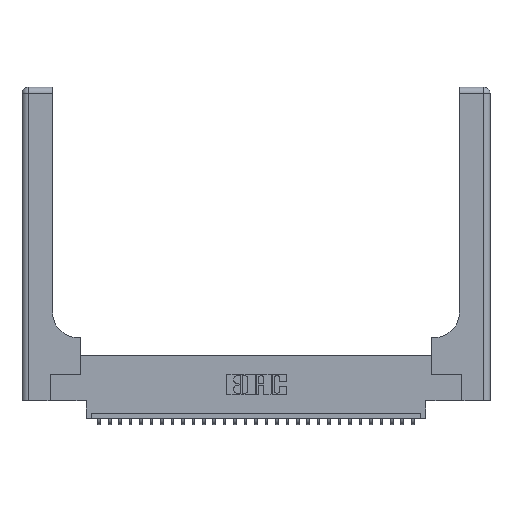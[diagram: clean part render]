
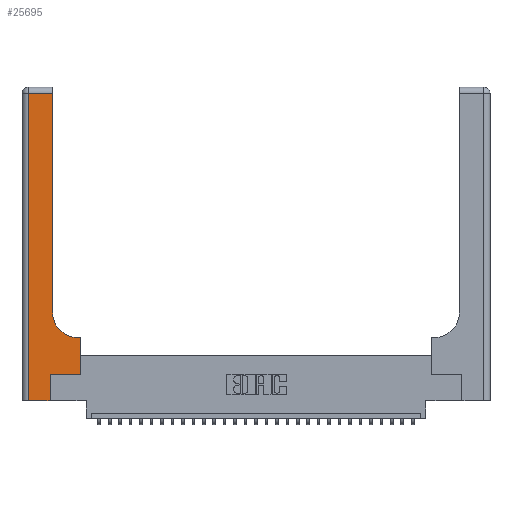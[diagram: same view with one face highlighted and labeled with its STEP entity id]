
A CAD part, top view. The second image highlights one B-rep face of the part: STEP entity #25695.
In plain terms, the highlighted planar face has unit normal (0, 0, 1).
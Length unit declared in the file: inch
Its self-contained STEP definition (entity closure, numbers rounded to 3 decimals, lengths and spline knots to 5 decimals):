
#50 = VERTEX_POINT ( 'NONE', #26670 ) ;
#305 = CARTESIAN_POINT ( 'NONE',  ( 0.5585, 0.6, 0.37 ) ) ;
#735 = LINE ( 'NONE', #1830, #29548 ) ;
#1077 = DIRECTION ( 'NONE',  ( -1., 0., 0. ) ) ;
#1157 = CARTESIAN_POINT ( 'NONE',  ( 0.269, 0., 0.37 ) ) ;
#1633 = CARTESIAN_POINT ( 'NONE',  ( 0.06, 3., 0.37 ) ) ;
#1830 = CARTESIAN_POINT ( 'NONE',  ( 0.2915, 3., 0.37 ) ) ;
#2615 = EDGE_CURVE ( 'NONE', #30106, #17821, #17179, .T. ) ;
#3046 = VERTEX_POINT ( 'NONE', #20566 ) ;
#3366 = LINE ( 'NONE', #15340, #21231 ) ;
#3525 = CARTESIAN_POINT ( 'NONE',  ( 0.2915, 0.85, 0.37 ) ) ;
#3790 = EDGE_CURVE ( 'NONE', #30160, #50, #735, .T. ) ;
#4427 = ORIENTED_EDGE ( 'NONE', *, *, #22223, .T. ) ;
#4945 = AXIS2_PLACEMENT_3D ( 'NONE', #26041, #18716, #7226 ) ;
#5159 = VECTOR ( 'NONE', #18166, 39.37008 ) ;
#5900 = DIRECTION ( 'NONE',  ( -1., 0., 0. ) ) ;
#6071 = DIRECTION ( 'NONE',  ( 0., 1., 0. ) ) ;
#6701 = CARTESIAN_POINT ( 'NONE',  ( 0.2915, 0.6, 0.37 ) ) ;
#6851 = ORIENTED_EDGE ( 'NONE', *, *, #26771, .T. ) ;
#7226 = DIRECTION ( 'NONE',  ( 1., 0., 0. ) ) ;
#7319 = ORIENTED_EDGE ( 'NONE', *, *, #2615, .T. ) ;
#7979 = VERTEX_POINT ( 'NONE', #305 ) ;
#8233 = CARTESIAN_POINT ( 'NONE',  ( 0.269, 0., 0.37 ) ) ;
#8283 = ORIENTED_EDGE ( 'NONE', *, *, #3790, .T. ) ;
#8446 = ORIENTED_EDGE ( 'NONE', *, *, #27316, .T. ) ;
#8536 = VERTEX_POINT ( 'NONE', #25619 ) ;
#8934 = CARTESIAN_POINT ( 'NONE',  ( 0.269, 0.25, 0.37 ) ) ;
#9036 = VECTOR ( 'NONE', #9052, 39.37008 ) ;
#9052 = DIRECTION ( 'NONE',  ( -1., 0., 0. ) ) ;
#10313 = EDGE_LOOP ( 'NONE', ( #8283, #11715, #18801, #7319, #12830, #27600, #8446, #4427, #6851 ) ) ;
#10820 = DIRECTION ( 'NONE',  ( 0., -1., 0. ) ) ;
#10860 = DIRECTION ( 'NONE',  ( 0., 1., 0. ) ) ;
#11262 = DIRECTION ( 'NONE',  ( 1., 0., 0. ) ) ;
#11715 = ORIENTED_EDGE ( 'NONE', *, *, #17148, .T. ) ;
#12176 = CIRCLE ( 'NONE', #4945, 0.25 ) ;
#12618 = VECTOR ( 'NONE', #10820, 39.37008 ) ;
#12830 = ORIENTED_EDGE ( 'NONE', *, *, #17544, .T. ) ;
#13718 = CARTESIAN_POINT ( 'NONE',  ( 0., 0., 0.37 ) ) ;
#14508 = LINE ( 'NONE', #6701, #9036 ) ;
#15340 = CARTESIAN_POINT ( 'NONE',  ( 0.5585, 0.25, 0.37 ) ) ;
#17043 = LINE ( 'NONE', #22276, #23590 ) ;
#17148 = EDGE_CURVE ( 'NONE', #50, #3046, #17043, .T. ) ;
#17179 = LINE ( 'NONE', #13718, #5159 ) ;
#17544 = EDGE_CURVE ( 'NONE', #17821, #8536, #24288, .T. ) ;
#17821 = VERTEX_POINT ( 'NONE', #8233 ) ;
#17862 = LINE ( 'NONE', #8934, #20074 ) ;
#18166 = DIRECTION ( 'NONE',  ( 1., 0., 0. ) ) ;
#18332 = EDGE_CURVE ( 'NONE', #3046, #30106, #18764, .T. ) ;
#18716 = DIRECTION ( 'NONE',  ( 0., 0., -1. ) ) ;
#18764 = LINE ( 'NONE', #1633, #12618 ) ;
#18801 = ORIENTED_EDGE ( 'NONE', *, *, #18332, .T. ) ;
#19918 = DIRECTION ( 'NONE',  ( 0., 0., -1. ) ) ;
#20074 = VECTOR ( 'NONE', #11262, 39.37008 ) ;
#20566 = CARTESIAN_POINT ( 'NONE',  ( 0.06, 2.94, 0.37 ) ) ;
#21231 = VECTOR ( 'NONE', #6071, 39.37008 ) ;
#21372 = CARTESIAN_POINT ( 'NONE',  ( 0.5415, 0.6, 0.37 ) ) ;
#22223 = EDGE_CURVE ( 'NONE', #7979, #24952, #14508, .T. ) ;
#22276 = CARTESIAN_POINT ( 'NONE',  ( 0., 2.94, 0.37 ) ) ;
#22971 = DIRECTION ( 'NONE',  ( 0., 1., 0. ) ) ;
#23590 = VECTOR ( 'NONE', #5900, 39.37008 ) ;
#24159 = CARTESIAN_POINT ( 'NONE',  ( 0.06, 0., 0.37 ) ) ;
#24288 = LINE ( 'NONE', #1157, #28706 ) ;
#24952 = VERTEX_POINT ( 'NONE', #21372 ) ;
#25084 = FACE_OUTER_BOUND ( 'NONE', #10313, .T. ) ;
#25619 = CARTESIAN_POINT ( 'NONE',  ( 0.269, 0.25, 0.37 ) ) ;
#25695 = ADVANCED_FACE ( 'NONE', ( #25084 ), #28897, .F. ) ;
#26002 = AXIS2_PLACEMENT_3D ( 'NONE', #26733, #19918, #1077 ) ;
#26041 = CARTESIAN_POINT ( 'NONE',  ( 0.5415, 0.85, 0.37 ) ) ;
#26076 = CARTESIAN_POINT ( 'NONE',  ( 0.5585, 0.25, 0.37 ) ) ;
#26251 = VERTEX_POINT ( 'NONE', #26076 ) ;
#26670 = CARTESIAN_POINT ( 'NONE',  ( 0.2915, 2.94, 0.37 ) ) ;
#26733 = CARTESIAN_POINT ( 'NONE',  ( 0., 3., 0.37 ) ) ;
#26771 = EDGE_CURVE ( 'NONE', #24952, #30160, #12176, .T. ) ;
#27316 = EDGE_CURVE ( 'NONE', #26251, #7979, #3366, .T. ) ;
#27600 = ORIENTED_EDGE ( 'NONE', *, *, #28717, .T. ) ;
#28706 = VECTOR ( 'NONE', #10860, 39.37008 ) ;
#28717 = EDGE_CURVE ( 'NONE', #8536, #26251, #17862, .T. ) ;
#28897 = PLANE ( 'NONE',  #26002 ) ;
#29548 = VECTOR ( 'NONE', #22971, 39.37008 ) ;
#30106 = VERTEX_POINT ( 'NONE', #24159 ) ;
#30160 = VERTEX_POINT ( 'NONE', #3525 ) ;
